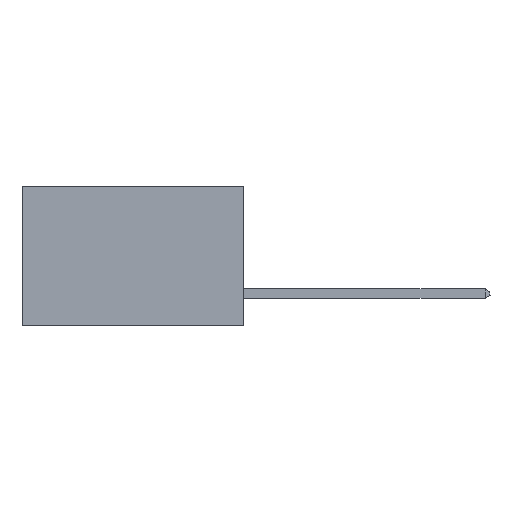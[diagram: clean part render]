
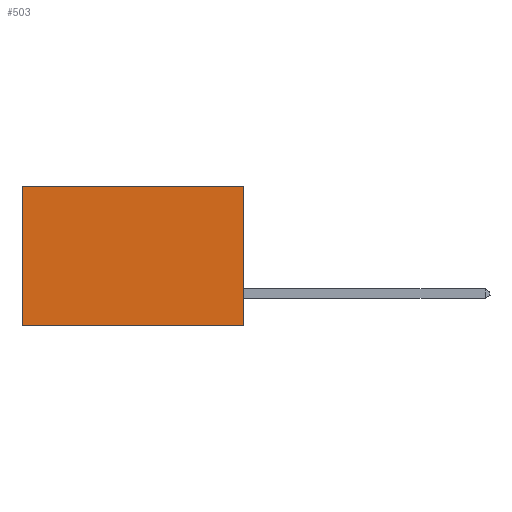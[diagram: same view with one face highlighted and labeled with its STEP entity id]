
A CAD part, left-side view. The second image highlights one B-rep face of the part: STEP entity #503.
In plain terms, the highlighted planar face has unit normal (-1, 0, 0).
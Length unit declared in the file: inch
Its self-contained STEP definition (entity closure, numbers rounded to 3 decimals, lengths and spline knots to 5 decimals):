
#503 = ADVANCED_FACE ( 'NONE', ( #20344 ), #12403, .F. ) ;
#1271 = VERTEX_POINT ( 'NONE', #24199 ) ;
#1430 = CARTESIAN_POINT ( 'NONE',  ( 0.277, 0., -0.37 ) ) ;
#3053 = EDGE_LOOP ( 'NONE', ( #13843, #22796, #23552, #28234 ) ) ;
#4711 = VERTEX_POINT ( 'NONE', #1430 ) ;
#5293 = DIRECTION ( 'NONE',  ( 1., 0., 0. ) ) ;
#7198 = CARTESIAN_POINT ( 'NONE',  ( 0.277, 0.59, 0. ) ) ;
#9551 = CARTESIAN_POINT ( 'NONE',  ( 0.277, 0., -0.37 ) ) ;
#9802 = DIRECTION ( 'NONE',  ( 0., 0., -1. ) ) ;
#10330 = DIRECTION ( 'NONE',  ( 0., 1., 0. ) ) ;
#12263 = LINE ( 'NONE', #29872, #23140 ) ;
#12403 = PLANE ( 'NONE',  #21967 ) ;
#13611 = DIRECTION ( 'NONE',  ( 0., 0., -1. ) ) ;
#13843 = ORIENTED_EDGE ( 'NONE', *, *, #17223, .T. ) ;
#15022 = VECTOR ( 'NONE', #10330, 39.37008 ) ;
#15428 = DIRECTION ( 'NONE',  ( 0., 1., 0. ) ) ;
#17223 = EDGE_CURVE ( 'NONE', #18706, #1271, #12263, .T. ) ;
#18706 = VERTEX_POINT ( 'NONE', #7198 ) ;
#19640 = CARTESIAN_POINT ( 'NONE',  ( 0.277, 0., 0. ) ) ;
#20344 = FACE_OUTER_BOUND ( 'NONE', #3053, .T. ) ;
#20696 = VERTEX_POINT ( 'NONE', #21521 ) ;
#20826 = LINE ( 'NONE', #22144, #26381 ) ;
#20884 = VECTOR ( 'NONE', #24656, 39.37008 ) ;
#21521 = CARTESIAN_POINT ( 'NONE',  ( 0.277, 0., 0. ) ) ;
#21632 = LINE ( 'NONE', #26944, #20884 ) ;
#21967 = AXIS2_PLACEMENT_3D ( 'NONE', #9551, #5293, #9802 ) ;
#22144 = CARTESIAN_POINT ( 'NONE',  ( 0.277, 0., -0.37 ) ) ;
#22464 = EDGE_CURVE ( 'NONE', #20696, #18706, #22578, .T. ) ;
#22578 = LINE ( 'NONE', #19640, #15022 ) ;
#22796 = ORIENTED_EDGE ( 'NONE', *, *, #28615, .F. ) ;
#23140 = VECTOR ( 'NONE', #13611, 39.37008 ) ;
#23552 = ORIENTED_EDGE ( 'NONE', *, *, #27755, .F. ) ;
#24199 = CARTESIAN_POINT ( 'NONE',  ( 0.277, 0.59, -0.37 ) ) ;
#24656 = DIRECTION ( 'NONE',  ( 0., 0., -1. ) ) ;
#26381 = VECTOR ( 'NONE', #15428, 39.37008 ) ;
#26944 = CARTESIAN_POINT ( 'NONE',  ( 0.277, 0., -0.37 ) ) ;
#27755 = EDGE_CURVE ( 'NONE', #20696, #4711, #21632, .T. ) ;
#28234 = ORIENTED_EDGE ( 'NONE', *, *, #22464, .T. ) ;
#28615 = EDGE_CURVE ( 'NONE', #4711, #1271, #20826, .T. ) ;
#29872 = CARTESIAN_POINT ( 'NONE',  ( 0.277, 0.59, -0.37 ) ) ;
